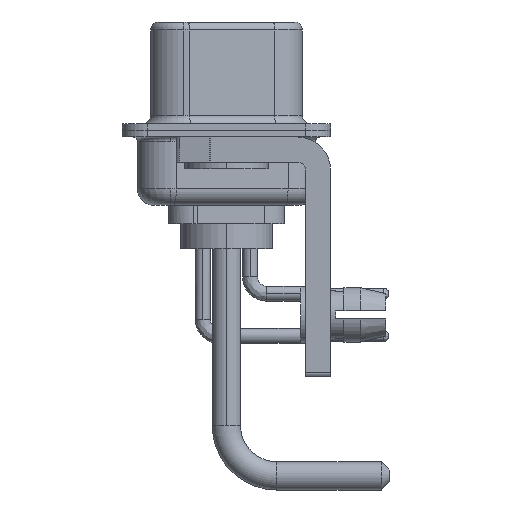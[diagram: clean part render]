
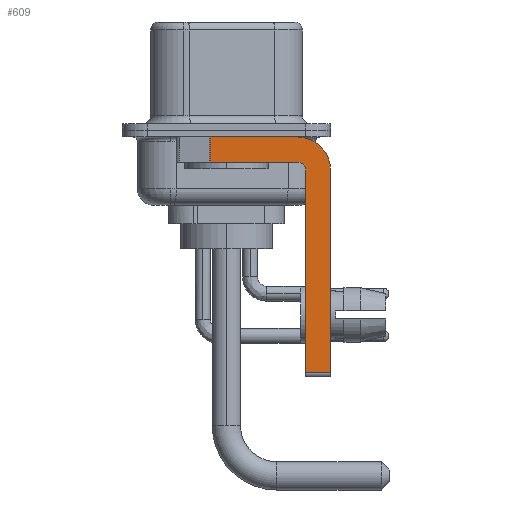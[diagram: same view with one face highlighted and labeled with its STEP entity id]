
A CAD part, left-side view. The second image highlights one B-rep face of the part: STEP entity #609.
In plain terms, the highlighted planar face has unit normal (-1, 0, 0).
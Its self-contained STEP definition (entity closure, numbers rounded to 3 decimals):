
#609 = ADVANCED_FACE ( 'NONE', ( #13370 ), #6173, .F. ) ;
#828 = DIRECTION ( 'NONE',  ( 1., 0., 0. ) ) ;
#1308 = ORIENTED_EDGE ( 'NONE', *, *, #3659, .F. ) ;
#1494 = DIRECTION ( 'NONE',  ( 1., 0., 0. ) ) ;
#1498 = ORIENTED_EDGE ( 'NONE', *, *, #20466, .F. ) ;
#2249 = EDGE_CURVE ( 'NONE', #19141, #16015, #5132, .T. ) ;
#2793 = CARTESIAN_POINT ( 'NONE',  ( -2.9, -4.25, -2.4 ) ) ;
#2838 = AXIS2_PLACEMENT_3D ( 'NONE', #29166, #3497, #12725 ) ;
#3183 = CARTESIAN_POINT ( 'NONE',  ( -2.9, -4.75, -14.8 ) ) ;
#3403 = ORIENTED_EDGE ( 'NONE', *, *, #26971, .F. ) ;
#3497 = DIRECTION ( 'NONE',  ( -1., 0., 0. ) ) ;
#3659 = EDGE_CURVE ( 'NONE', #7724, #30163, #6081, .T. ) ;
#3981 = DIRECTION ( 'NONE',  ( 0., 0., -1. ) ) ;
#4084 = LINE ( 'NONE', #27899, #14197 ) ;
#4164 = EDGE_CURVE ( 'NONE', #19188, #16983, #15055, .T. ) ;
#4203 = CARTESIAN_POINT ( 'NONE',  ( -2.9, -6.25, -2.4 ) ) ;
#5132 = LINE ( 'NONE', #26423, #20930 ) ;
#5720 = CARTESIAN_POINT ( 'NONE',  ( -2.9, -4.25, -2.4 ) ) ;
#6081 = CIRCLE ( 'NONE', #27060, 2. ) ;
#6173 = PLANE ( 'NONE',  #16354 ) ;
#7386 = CARTESIAN_POINT ( 'NONE',  ( -2.9, -4.25, -1.9 ) ) ;
#7724 = VERTEX_POINT ( 'NONE', #9687 ) ;
#7850 = VERTEX_POINT ( 'NONE', #15534 ) ;
#9546 = ORIENTED_EDGE ( 'NONE', *, *, #24501, .F. ) ;
#9687 = CARTESIAN_POINT ( 'NONE',  ( -2.9, -4.25, -0.4 ) ) ;
#10873 = ORIENTED_EDGE ( 'NONE', *, *, #4164, .F. ) ;
#11110 = VECTOR ( 'NONE', #16574, 1000. ) ;
#11327 = LINE ( 'NONE', #21151, #13216 ) ;
#11409 = ORIENTED_EDGE ( 'NONE', *, *, #2249, .T. ) ;
#12725 = DIRECTION ( 'NONE',  ( 0., 0., 1. ) ) ;
#13216 = VECTOR ( 'NONE', #17051, 1000. ) ;
#13370 = FACE_OUTER_BOUND ( 'NONE', #17268, .T. ) ;
#13578 = LINE ( 'NONE', #23592, #29843 ) ;
#14197 = VECTOR ( 'NONE', #25515, 1000. ) ;
#14658 = DIRECTION ( 'NONE',  ( 0., 0., -1. ) ) ;
#15055 = LINE ( 'NONE', #3183, #16859 ) ;
#15522 = EDGE_CURVE ( 'NONE', #27700, #16015, #23797, .T. ) ;
#15534 = CARTESIAN_POINT ( 'NONE',  ( -2.9, -6.25, -14.55 ) ) ;
#16015 = VERTEX_POINT ( 'NONE', #21886 ) ;
#16354 = AXIS2_PLACEMENT_3D ( 'NONE', #5720, #1494, #3981 ) ;
#16541 = DIRECTION ( 'NONE',  ( 0., 0., -1. ) ) ;
#16574 = DIRECTION ( 'NONE',  ( 0., 1., 0. ) ) ;
#16859 = VECTOR ( 'NONE', #17253, 1000. ) ;
#16983 = VERTEX_POINT ( 'NONE', #28025 ) ;
#17051 = DIRECTION ( 'NONE',  ( 0., -1., 0. ) ) ;
#17253 = DIRECTION ( 'NONE',  ( 0., 0., 1. ) ) ;
#17268 = EDGE_LOOP ( 'NONE', ( #9546, #11409, #20544, #1498, #10873, #23370, #3403, #1308 ) ) ;
#19141 = VERTEX_POINT ( 'NONE', #26352 ) ;
#19188 = VERTEX_POINT ( 'NONE', #21957 ) ;
#20242 = CARTESIAN_POINT ( 'NONE',  ( -2.9, -4.25, -1.9 ) ) ;
#20466 = EDGE_CURVE ( 'NONE', #16983, #27700, #27852, .T. ) ;
#20544 = ORIENTED_EDGE ( 'NONE', *, *, #15522, .F. ) ;
#20930 = VECTOR ( 'NONE', #14658, 1000. ) ;
#20942 = DIRECTION ( 'NONE',  ( 0., 0., -1. ) ) ;
#21151 = CARTESIAN_POINT ( 'NONE',  ( -2.9, -4.25, -14.55 ) ) ;
#21886 = CARTESIAN_POINT ( 'NONE',  ( -2.9, 0.978, -1.9 ) ) ;
#21957 = CARTESIAN_POINT ( 'NONE',  ( -2.9, -4.75, -14.55 ) ) ;
#23370 = ORIENTED_EDGE ( 'NONE', *, *, #24808, .T. ) ;
#23592 = CARTESIAN_POINT ( 'NONE',  ( -2.9, -6.25, -2.4 ) ) ;
#23797 = LINE ( 'NONE', #7386, #11110 ) ;
#24501 = EDGE_CURVE ( 'NONE', #19141, #7724, #4084, .T. ) ;
#24808 = EDGE_CURVE ( 'NONE', #19188, #7850, #11327, .T. ) ;
#25515 = DIRECTION ( 'NONE',  ( 0., -1., 0. ) ) ;
#26352 = CARTESIAN_POINT ( 'NONE',  ( -2.9, 0.978, -0.4 ) ) ;
#26423 = CARTESIAN_POINT ( 'NONE',  ( -2.9, 0.978, -1.9 ) ) ;
#26971 = EDGE_CURVE ( 'NONE', #30163, #7850, #13578, .T. ) ;
#27060 = AXIS2_PLACEMENT_3D ( 'NONE', #2793, #828, #16541 ) ;
#27700 = VERTEX_POINT ( 'NONE', #20242 ) ;
#27852 = CIRCLE ( 'NONE', #2838, 0.5 ) ;
#27899 = CARTESIAN_POINT ( 'NONE',  ( -2.9, 3., -0.4 ) ) ;
#28025 = CARTESIAN_POINT ( 'NONE',  ( -2.9, -4.75, -2.4 ) ) ;
#29166 = CARTESIAN_POINT ( 'NONE',  ( -2.9, -4.25, -2.4 ) ) ;
#29843 = VECTOR ( 'NONE', #20942, 1000. ) ;
#30163 = VERTEX_POINT ( 'NONE', #4203 ) ;
